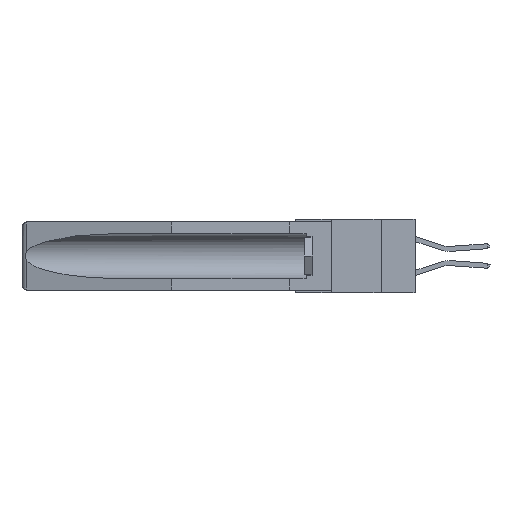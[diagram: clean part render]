
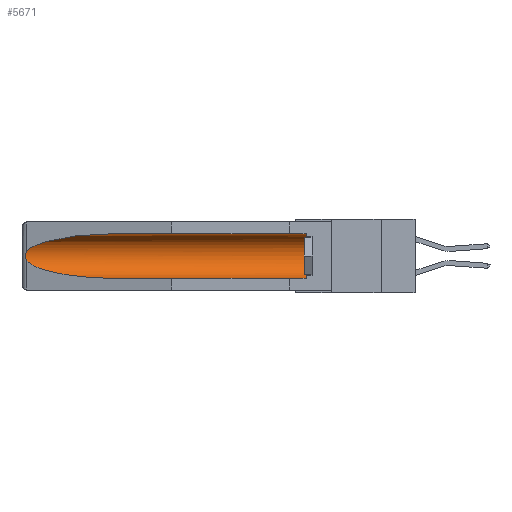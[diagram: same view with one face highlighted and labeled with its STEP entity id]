
A CAD part, left-side view. The second image highlights one B-rep face of the part: STEP entity #5671.
In plain terms, the highlighted cylindrical face has radius 2.857 mm (diameter 5.715 mm), a partial arc.
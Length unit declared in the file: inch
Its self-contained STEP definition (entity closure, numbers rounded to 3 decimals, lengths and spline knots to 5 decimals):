
#17 = VECTOR ( 'NONE', #8693, 39.37008 ) ;
#183 = EDGE_CURVE ( 'NONE', #1389, #17316, #4742, .T. ) ;
#426 = CARTESIAN_POINT ( 'NONE',  ( 0.155, 1.07973, -0.284 ) ) ;
#1175 = CARTESIAN_POINT ( 'NONE',  ( 0.21114, 1.30732, -0.059 ) ) ;
#1389 = VERTEX_POINT ( 'NONE', #20223 ) ;
#1649 = CARTESIAN_POINT ( 'NONE',  ( 0.26537, 1.52718, -0.19328 ) ) ;
#2007 = CARTESIAN_POINT ( 'NONE',  ( 0.26537, 1.52718, -0.19328 ) ) ;
#2106 = CARTESIAN_POINT ( 'NONE',  ( 0.26597, 1.5296, -0.19026 ) ) ;
#2357 = VERTEX_POINT ( 'NONE', #9073 ) ;
#2581 = DIRECTION ( 'NONE',  ( 0., -1., 0. ) ) ;
#3921 = CARTESIAN_POINT ( 'NONE',  ( 0.26597, 1.52961, -0.15275 ) ) ;
#4541 = CARTESIAN_POINT ( 'NONE',  ( 0.155, -0.30754, -0.059 ) ) ;
#4742 = B_SPLINE_CURVE_WITH_KNOTS ( 'NONE', 3,
 ( #22978, #3921, #21393, #5849, #17235, #19358, #21312, #13607, #2106, #9717 ),
 .UNSPECIFIED., .F., .F.,
 ( 4, 2, 2, 2, 4 ),
 ( 0., 0.00029, 0.00058, 0.00087, 0.00117 ),
 .UNSPECIFIED. ) ;
#5318 = AXIS2_PLACEMENT_3D ( 'NONE', #18004, #2581, #24027 ) ;
#5671 = ADVANCED_FACE ( 'NONE', ( #17144 ), #12035, .F. ) ;
#5849 = CARTESIAN_POINT ( 'NONE',  ( 0.2673, 1.5327, -0.16383 ) ) ;
#7651 = DIRECTION ( 'NONE',  ( 0., 0., 1. ) ) ;
#8138 =( BOUNDED_CURVE ( )  B_SPLINE_CURVE ( 3, ( #22212, #1175, #8877, #18423 ),
 .UNSPECIFIED., .F., .F. ) 
 B_SPLINE_CURVE_WITH_KNOTS ( ( 4, 4 ),
 ( 4.71239, 6.08839 ),
 .UNSPECIFIED. ) 
 CURVE ( )  GEOMETRIC_REPRESENTATION_ITEM ( )  RATIONAL_B_SPLINE_CURVE ( ( 1., 0.848, 0.848, 1. ) ) 
 REPRESENTATION_ITEM ( '' )  );
#8194 = EDGE_CURVE ( 'NONE', #9918, #2357, #12027, .T. ) ;
#8693 = DIRECTION ( 'NONE',  ( 0., 1., 0. ) ) ;
#8877 = CARTESIAN_POINT ( 'NONE',  ( 0.25451, 1.48313, -0.09465 ) ) ;
#9073 = CARTESIAN_POINT ( 'NONE',  ( 0.155, 1.07973, -0.059 ) ) ;
#9221 = ORIENTED_EDGE ( 'NONE', *, *, #13740, .T. ) ;
#9301 = LINE ( 'NONE', #10882, #17 ) ;
#9391 = CARTESIAN_POINT ( 'NONE',  ( 0.155, 0.126, -0.284 ) ) ;
#9717 = CARTESIAN_POINT ( 'NONE',  ( 0.26537, 1.52718, -0.19328 ) ) ;
#9918 = VERTEX_POINT ( 'NONE', #20573 ) ;
#10882 = CARTESIAN_POINT ( 'NONE',  ( 0.155, -0.30754, -0.284 ) ) ;
#12000 = EDGE_CURVE ( 'NONE', #2357, #1389, #8138, .T. ) ;
#12027 = LINE ( 'NONE', #4541, #15019 ) ;
#12035 = CYLINDRICAL_SURFACE ( 'NONE', #17727, 0.1125 ) ;
#12325 = CARTESIAN_POINT ( 'NONE',  ( 0.155, 1.07973, -0.284 ) ) ;
#13607 = CARTESIAN_POINT ( 'NONE',  ( 0.26655, 1.53094, -0.18657 ) ) ;
#13740 = EDGE_CURVE ( 'NONE', #21065, #9918, #16684, .T. ) ;
#14690 = ORIENTED_EDGE ( 'NONE', *, *, #8194, .T. ) ;
#15019 = VECTOR ( 'NONE', #18123, 39.37008 ) ;
#15161 = ORIENTED_EDGE ( 'NONE', *, *, #16358, .F. ) ;
#15189 = CARTESIAN_POINT ( 'NONE',  ( 0.21114, 1.30732, -0.284 ) ) ;
#15341 = CARTESIAN_POINT ( 'NONE',  ( 0.155, -0.30754, -0.1715 ) ) ;
#16187 = VERTEX_POINT ( 'NONE', #12325 ) ;
#16358 = EDGE_CURVE ( 'NONE', #21065, #16187, #9301, .T. ) ;
#16684 = CIRCLE ( 'NONE', #5318, 0.1125 ) ;
#17144 = FACE_OUTER_BOUND ( 'NONE', #23028, .T. ) ;
#17235 = CARTESIAN_POINT ( 'NONE',  ( 0.2675, 1.53308, -0.16763 ) ) ;
#17316 = VERTEX_POINT ( 'NONE', #1649 ) ;
#17409 = CARTESIAN_POINT ( 'NONE',  ( 0.25451, 1.48313, -0.24835 ) ) ;
#17727 = AXIS2_PLACEMENT_3D ( 'NONE', #15341, #21100, #7651 ) ;
#18004 = CARTESIAN_POINT ( 'NONE',  ( 0.155, 0.126, -0.1715 ) ) ;
#18123 = DIRECTION ( 'NONE',  ( 0., 1., 0. ) ) ;
#18423 = CARTESIAN_POINT ( 'NONE',  ( 0.26537, 1.52718, -0.14972 ) ) ;
#19358 = CARTESIAN_POINT ( 'NONE',  ( 0.2675, 1.53308, -0.17534 ) ) ;
#20223 = CARTESIAN_POINT ( 'NONE',  ( 0.26537, 1.52718, -0.14972 ) ) ;
#20349 = EDGE_CURVE ( 'NONE', #17316, #16187, #23465, .T. ) ;
#20573 = CARTESIAN_POINT ( 'NONE',  ( 0.155, 0.126, -0.059 ) ) ;
#21065 = VERTEX_POINT ( 'NONE', #9391 ) ;
#21100 = DIRECTION ( 'NONE',  ( 0., 1., 0. ) ) ;
#21277 = ORIENTED_EDGE ( 'NONE', *, *, #20349, .T. ) ;
#21312 = CARTESIAN_POINT ( 'NONE',  ( 0.2673, 1.53269, -0.17917 ) ) ;
#21393 = CARTESIAN_POINT ( 'NONE',  ( 0.26654, 1.53092, -0.15636 ) ) ;
#22212 = CARTESIAN_POINT ( 'NONE',  ( 0.155, 1.07973, -0.059 ) ) ;
#22786 = ORIENTED_EDGE ( 'NONE', *, *, #183, .T. ) ;
#22978 = CARTESIAN_POINT ( 'NONE',  ( 0.26537, 1.52718, -0.14972 ) ) ;
#23028 = EDGE_LOOP ( 'NONE', ( #24736, #22786, #21277, #15161, #9221, #14690 ) ) ;
#23465 =( BOUNDED_CURVE ( )  B_SPLINE_CURVE ( 3, ( #2007, #17409, #15189, #426 ),
 .UNSPECIFIED., .F., .F. ) 
 B_SPLINE_CURVE_WITH_KNOTS ( ( 4, 4 ),
 ( 0.1948, 1.5708 ),
 .UNSPECIFIED. ) 
 CURVE ( )  GEOMETRIC_REPRESENTATION_ITEM ( )  RATIONAL_B_SPLINE_CURVE ( ( 1., 0.848, 0.848, 1. ) ) 
 REPRESENTATION_ITEM ( '' )  );
#24027 = DIRECTION ( 'NONE',  ( 0., 0., 1. ) ) ;
#24736 = ORIENTED_EDGE ( 'NONE', *, *, #12000, .T. ) ;
